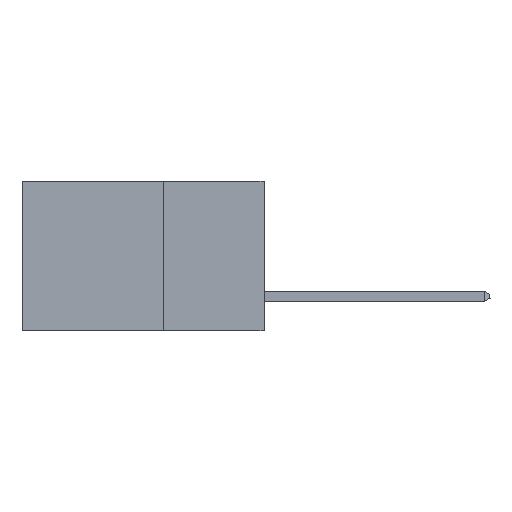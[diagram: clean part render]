
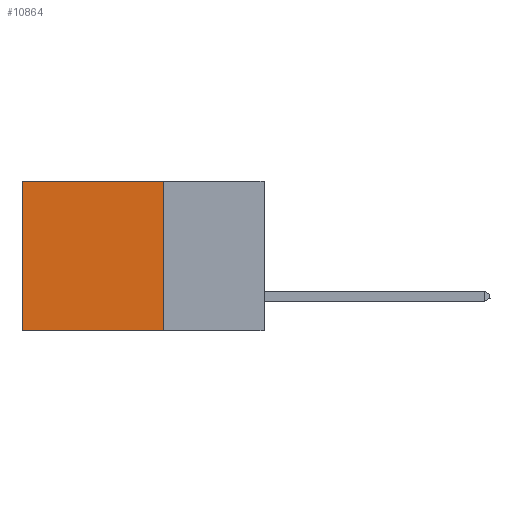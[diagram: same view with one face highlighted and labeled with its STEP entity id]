
A CAD part, left-side view. The second image highlights one B-rep face of the part: STEP entity #10864.
In plain terms, the highlighted planar face has unit normal (-1, 0, 0).
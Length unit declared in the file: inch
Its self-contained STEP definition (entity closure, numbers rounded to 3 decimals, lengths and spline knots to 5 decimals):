
#1115 = CARTESIAN_POINT ( 'NONE',  ( 0.298, 0.25, 0. ) ) ;
#1745 = VECTOR ( 'NONE', #4698, 39.37008 ) ;
#3151 = CARTESIAN_POINT ( 'NONE',  ( 0.298, 0.6, 0. ) ) ;
#4037 = EDGE_CURVE ( 'NONE', #28888, #22426, #20028, .T. ) ;
#4408 = CARTESIAN_POINT ( 'NONE',  ( 0.298, 0.25, -0.37 ) ) ;
#4698 = DIRECTION ( 'NONE',  ( 0., 0., -1. ) ) ;
#5417 = LINE ( 'NONE', #3151, #16807 ) ;
#5505 = DIRECTION ( 'NONE',  ( 0., 0., -1. ) ) ;
#5802 = ORIENTED_EDGE ( 'NONE', *, *, #11215, .T. ) ;
#5832 = CARTESIAN_POINT ( 'NONE',  ( 0.298, 0.25, 0. ) ) ;
#7077 = CARTESIAN_POINT ( 'NONE',  ( 0.298, 0.6, -0.37 ) ) ;
#7979 = CARTESIAN_POINT ( 'NONE',  ( 0.298, 0.6, 0. ) ) ;
#8591 = ORIENTED_EDGE ( 'NONE', *, *, #22818, .T. ) ;
#8646 = PLANE ( 'NONE',  #17440 ) ;
#9937 = VERTEX_POINT ( 'NONE', #7979 ) ;
#10183 = LINE ( 'NONE', #22867, #28078 ) ;
#10530 = VERTEX_POINT ( 'NONE', #7077 ) ;
#10864 = ADVANCED_FACE ( 'NONE', ( #22883 ), #8646, .F. ) ;
#11215 = EDGE_CURVE ( 'NONE', #9937, #10530, #5417, .T. ) ;
#13140 = VECTOR ( 'NONE', #23976, 39.37008 ) ;
#13156 = DIRECTION ( 'NONE',  ( 1., 0., 0. ) ) ;
#13696 = DIRECTION ( 'NONE',  ( 0., 1., 0. ) ) ;
#14548 = LINE ( 'NONE', #5832, #13140 ) ;
#16807 = VECTOR ( 'NONE', #5505, 39.37008 ) ;
#17440 = AXIS2_PLACEMENT_3D ( 'NONE', #24460, #13156, #28825 ) ;
#17770 = CARTESIAN_POINT ( 'NONE',  ( 0.298, 0.25, 0. ) ) ;
#20028 = LINE ( 'NONE', #17770, #1745 ) ;
#20078 = ORIENTED_EDGE ( 'NONE', *, *, #4037, .F. ) ;
#21993 = EDGE_LOOP ( 'NONE', ( #5802, #25197, #20078, #8591 ) ) ;
#22426 = VERTEX_POINT ( 'NONE', #4408 ) ;
#22818 = EDGE_CURVE ( 'NONE', #28888, #9937, #14548, .T. ) ;
#22867 = CARTESIAN_POINT ( 'NONE',  ( 0.298, 0.25, -0.37 ) ) ;
#22883 = FACE_OUTER_BOUND ( 'NONE', #21993, .T. ) ;
#23976 = DIRECTION ( 'NONE',  ( 0., 1., 0. ) ) ;
#24460 = CARTESIAN_POINT ( 'NONE',  ( 0.298, 0.25, 0. ) ) ;
#25197 = ORIENTED_EDGE ( 'NONE', *, *, #25995, .F. ) ;
#25995 = EDGE_CURVE ( 'NONE', #22426, #10530, #10183, .T. ) ;
#28078 = VECTOR ( 'NONE', #13696, 39.37008 ) ;
#28825 = DIRECTION ( 'NONE',  ( 0., 0., -1. ) ) ;
#28888 = VERTEX_POINT ( 'NONE', #1115 ) ;
